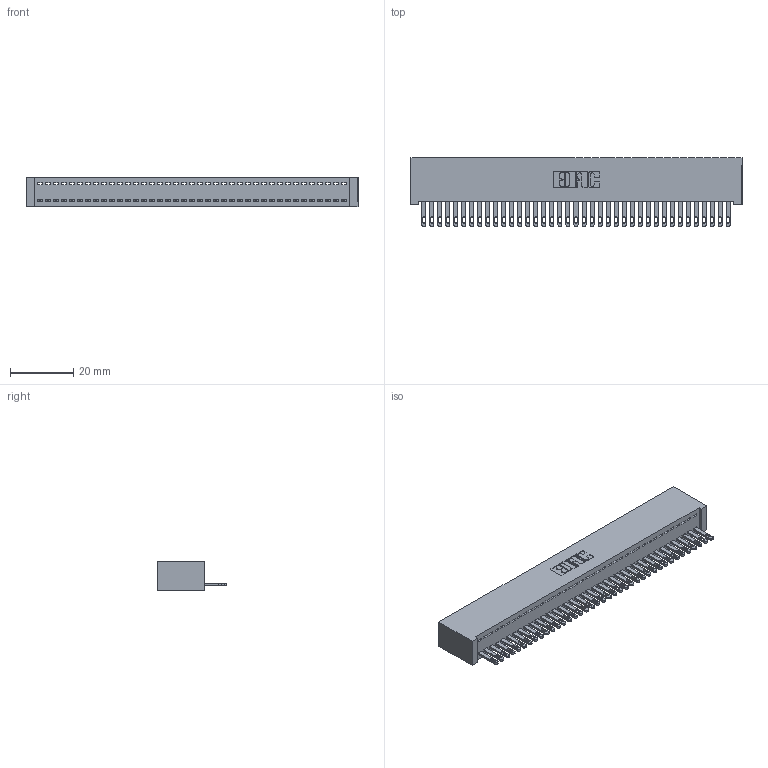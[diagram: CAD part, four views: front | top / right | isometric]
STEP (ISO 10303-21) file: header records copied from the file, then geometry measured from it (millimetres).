
FILE_DESCRIPTION (( 'STEP AP203' ), '1' );
FILE_NAME ('892-039-500-101.STEP', '2020-09-21T16:15:49', ( '' ), ( '' ), 'SwSTEP 2.0', 'SolidWorks 2020', '' );
FILE_SCHEMA (( 'CONFIG_CONTROL_DESIGN' ));
Length unit declared in the file: inch
Products named in the file (3): 842 Part_Lugless; 345-292-001_345-293-100; 892-039-500-101
Assembly tree (40 placements, depth 2):
  892-039-500-101
    842 Part_Lugless
    345-292-001_345-293-100  x39
Bounding box: 105.31 x 21.85 x 9.4 mm (x, y, z)
Volume: 9655.5 mm3; surface area: 14522.7 mm2
Topology: 40 solids, 40 shells, 2208 faces, 6827 edges, 4550 vertices
Faces by surface type: plane 1466, cylinder 742
Entity records: 23751 total; most frequent: CARTESIAN_POINT 4103, ORIENTED_EDGE 4078, DIRECTION 3461, EDGE_CURVE 2039, VECTOR 1915, LINE 1915, VERTEX_POINT 1358, AXIS2_PLACEMENT_3D 773
